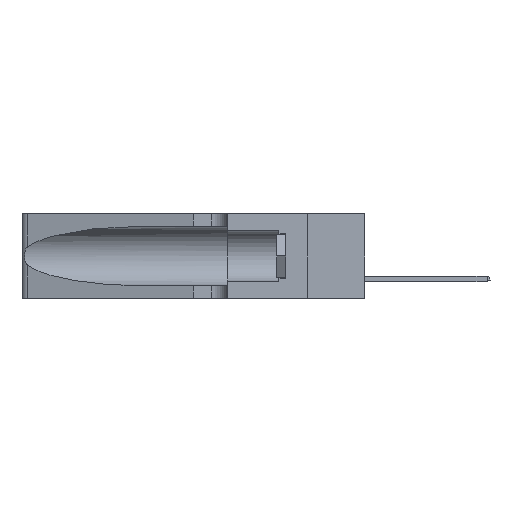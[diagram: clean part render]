
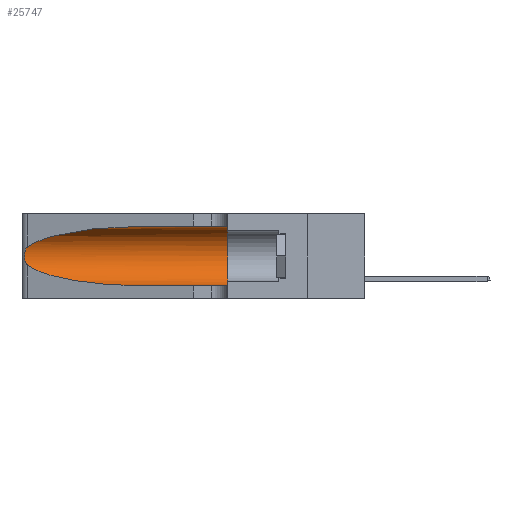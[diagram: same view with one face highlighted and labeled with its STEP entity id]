
A CAD part, left-side view. The second image highlights one B-rep face of the part: STEP entity #25747.
In plain terms, the highlighted cylindrical face has radius 3.308 mm (diameter 6.617 mm), a partial arc.
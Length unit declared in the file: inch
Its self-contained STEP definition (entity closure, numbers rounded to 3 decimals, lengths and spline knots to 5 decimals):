
#19 = CYLINDRICAL_SURFACE ( 'NONE', #30055, 0.13025 ) ;
#335 = ORIENTED_EDGE ( 'NONE', *, *, #33862, .T. ) ;
#600 = CARTESIAN_POINT ( 'NONE',  ( 0.18966, 0.96281, 0.31525 ) ) ;
#1513 = CARTESIAN_POINT ( 'NONE',  ( 0.1305, 0.72297, 0.31525 ) ) ;
#3760 = CARTESIAN_POINT ( 'NONE',  ( 0.26075, 1.23896, 0.19203 ) ) ;
#3818 = EDGE_CURVE ( 'NONE', #25705, #20161, #23223, .T. ) ;
#4036 = CARTESIAN_POINT ( 'NONE',  ( 0.25856, 1.23593, 0.16098 ) ) ;
#5105 = AXIS2_PLACEMENT_3D ( 'NONE', #30330, #15259, #8799 ) ;
#5111 = CARTESIAN_POINT ( 'NONE',  ( 0.1305, 0.35, 0.05475 ) ) ;
#5818 = DIRECTION ( 'NONE',  ( 0., -1., 0. ) ) ;
#6645 = VERTEX_POINT ( 'NONE', #17112 ) ;
#6914 =( BOUNDED_CURVE ( )  B_SPLINE_CURVE ( 3, ( #20036, #11401, #32174, #8342 ),
 .UNSPECIFIED., .F., .F. ) 
 B_SPLINE_CURVE_WITH_KNOTS ( ( 4, 4 ),
 ( 3.44316, 4.71239 ),
 .UNSPECIFIED. ) 
 CURVE ( )  GEOMETRIC_REPRESENTATION_ITEM ( )  RATIONAL_B_SPLINE_CURVE ( ( 1., 0.87, 0.87, 1. ) ) 
 REPRESENTATION_ITEM ( '' )  );
#7173 = CARTESIAN_POINT ( 'NONE',  ( 0.1305, 1.61858, 0.185 ) ) ;
#7423 = LINE ( 'NONE', #27235, #29741 ) ;
#8342 = CARTESIAN_POINT ( 'NONE',  ( 0.1305, 0.72297, 0.05475 ) ) ;
#8799 = DIRECTION ( 'NONE',  ( 0., 0., 1. ) ) ;
#9360 =( BOUNDED_CURVE ( )  B_SPLINE_CURVE ( 3, ( #34476, #600, #24949, #38261 ),
 .UNSPECIFIED., .F., .T. ) 
 B_SPLINE_CURVE_WITH_KNOTS ( ( 4, 4 ),
 ( 1.5708, 2.84003 ),
 .UNSPECIFIED. ) 
 CURVE ( )  GEOMETRIC_REPRESENTATION_ITEM ( )  RATIONAL_B_SPLINE_CURVE ( ( 1., 0.87, 0.87, 1. ) ) 
 REPRESENTATION_ITEM ( '' )  );
#10310 = CARTESIAN_POINT ( 'NONE',  ( 0.25639, 1.23186, 0.15144 ) ) ;
#11401 = CARTESIAN_POINT ( 'NONE',  ( 0.2373, 1.15595, 0.08982 ) ) ;
#11806 = DIRECTION ( 'NONE',  ( 0., -1., 0. ) ) ;
#12192 = ORIENTED_EDGE ( 'NONE', *, *, #35628, .T. ) ;
#12566 = ORIENTED_EDGE ( 'NONE', *, *, #21627, .F. ) ;
#12946 = VERTEX_POINT ( 'NONE', #19727 ) ;
#13106 = CARTESIAN_POINT ( 'NONE',  ( 0.25555, 1.22993, 0.14849 ) ) ;
#15106 = CARTESIAN_POINT ( 'NONE',  ( 0.1305, 1.61858, 0.31525 ) ) ;
#15259 = DIRECTION ( 'NONE',  ( 0., 1., 0. ) ) ;
#15960 = EDGE_CURVE ( 'NONE', #6645, #12946, #38636, .T. ) ;
#16415 = CARTESIAN_POINT ( 'NONE',  ( 0.25789, 1.23486, 0.15765 ) ) ;
#16614 = VERTEX_POINT ( 'NONE', #36182 ) ;
#16767 = ORIENTED_EDGE ( 'NONE', *, *, #19847, .T. ) ;
#16898 = LINE ( 'NONE', #15106, #39211 ) ;
#17112 = CARTESIAN_POINT ( 'NONE',  ( 0.25487, 1.22718, 0.22369 ) ) ;
#17737 = ORIENTED_EDGE ( 'NONE', *, *, #3818, .F. ) ;
#17820 = FACE_OUTER_BOUND ( 'NONE', #35384, .T. ) ;
#19727 = CARTESIAN_POINT ( 'NONE',  ( 0.25487, 1.22718, 0.14631 ) ) ;
#19847 = EDGE_CURVE ( 'NONE', #23547, #6645, #9360, .T. ) ;
#19977 = DIRECTION ( 'NONE',  ( 0., -1., 0. ) ) ;
#20036 = CARTESIAN_POINT ( 'NONE',  ( 0.25487, 1.22718, 0.14631 ) ) ;
#20161 = VERTEX_POINT ( 'NONE', #5111 ) ;
#21627 = EDGE_CURVE ( 'NONE', #23547, #25705, #16898, .T. ) ;
#22112 = CARTESIAN_POINT ( 'NONE',  ( 0.25787, 1.23484, 0.2124 ) ) ;
#22604 = DIRECTION ( 'NONE',  ( 0., 0., -1. ) ) ;
#23223 = CIRCLE ( 'NONE', #5105, 0.13025 ) ;
#23547 = VERTEX_POINT ( 'NONE', #1513 ) ;
#24949 = CARTESIAN_POINT ( 'NONE',  ( 0.2373, 1.15595, 0.28018 ) ) ;
#25148 = CARTESIAN_POINT ( 'NONE',  ( 0.25555, 1.22994, 0.2215 ) ) ;
#25350 = CARTESIAN_POINT ( 'NONE',  ( 0.1305, 0.35, 0.31525 ) ) ;
#25705 = VERTEX_POINT ( 'NONE', #25350 ) ;
#25747 = ADVANCED_FACE ( 'NONE', ( #17820 ), #19, .F. ) ;
#27235 = CARTESIAN_POINT ( 'NONE',  ( 0.1305, 1.61858, 0.05475 ) ) ;
#28425 = CARTESIAN_POINT ( 'NONE',  ( 0.26075, 1.23896, 0.178 ) ) ;
#29741 = VECTOR ( 'NONE', #5818, 39.37008 ) ;
#30055 = AXIS2_PLACEMENT_3D ( 'NONE', #7173, #19977, #22604 ) ;
#30330 = CARTESIAN_POINT ( 'NONE',  ( 0.1305, 0.35, 0.185 ) ) ;
#31080 = CARTESIAN_POINT ( 'NONE',  ( 0.25639, 1.23184, 0.21858 ) ) ;
#31504 = CARTESIAN_POINT ( 'NONE',  ( 0.25487, 1.22718, 0.14631 ) ) ;
#32174 = CARTESIAN_POINT ( 'NONE',  ( 0.18966, 0.96281, 0.05475 ) ) ;
#33862 = EDGE_CURVE ( 'NONE', #16614, #20161, #7423, .T. ) ;
#34179 = CARTESIAN_POINT ( 'NONE',  ( 0.25487, 1.22718, 0.22369 ) ) ;
#34476 = CARTESIAN_POINT ( 'NONE',  ( 0.1305, 0.72297, 0.31525 ) ) ;
#34590 = CARTESIAN_POINT ( 'NONE',  ( 0.26017, 1.23833, 0.17102 ) ) ;
#35384 = EDGE_LOOP ( 'NONE', ( #16767, #35783, #12192, #335, #17737, #12566 ) ) ;
#35628 = EDGE_CURVE ( 'NONE', #12946, #16614, #6914, .T. ) ;
#35783 = ORIENTED_EDGE ( 'NONE', *, *, #15960, .T. ) ;
#36182 = CARTESIAN_POINT ( 'NONE',  ( 0.1305, 0.72297, 0.05475 ) ) ;
#37076 = CARTESIAN_POINT ( 'NONE',  ( 0.26018, 1.23835, 0.19895 ) ) ;
#37498 = CARTESIAN_POINT ( 'NONE',  ( 0.25854, 1.2359, 0.20912 ) ) ;
#38261 = CARTESIAN_POINT ( 'NONE',  ( 0.25487, 1.22718, 0.22369 ) ) ;
#38636 = B_SPLINE_CURVE_WITH_KNOTS ( 'NONE', 3,
 ( #34179, #25148, #31080, #22112, #37498, #37076, #3760, #28425, #34590, #4036, #16415, #10310, #13106, #31504 ),
 .UNSPECIFIED., .F., .F.,
 ( 4, 2, 2, 2, 2, 2, 4 ),
 ( 0., 0.00027, 0.00053, 0.00107, 0.0016, 0.00187, 0.00214 ),
 .UNSPECIFIED. ) ;
#39211 = VECTOR ( 'NONE', #11806, 39.37008 ) ;
